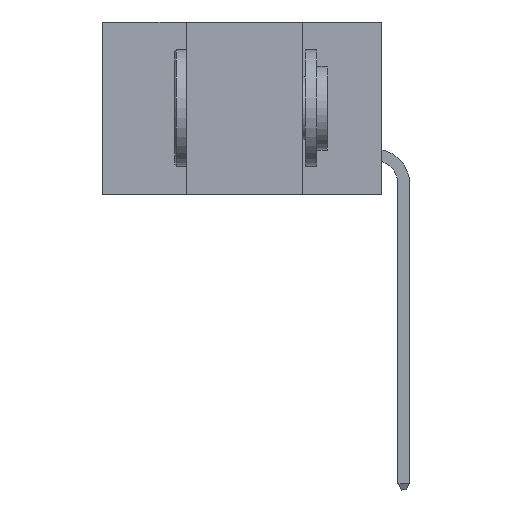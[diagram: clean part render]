
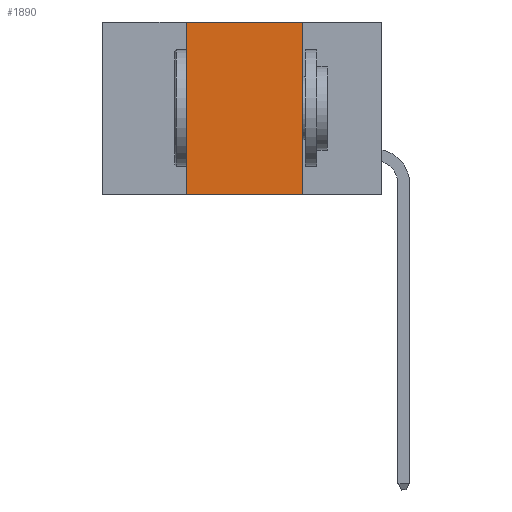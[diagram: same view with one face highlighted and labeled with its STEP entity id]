
A CAD part, left-side view. The second image highlights one B-rep face of the part: STEP entity #1890.
In plain terms, the highlighted planar face has unit normal (-1, 0, 0).
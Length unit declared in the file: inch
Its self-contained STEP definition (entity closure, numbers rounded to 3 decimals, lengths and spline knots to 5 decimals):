
#1890 = ADVANCED_FACE ( 'NONE', ( #22624 ), #2279, .F. ) ;
#2071 = EDGE_CURVE ( 'NONE', #20057, #4016, #4633, .T. ) ;
#2279 = PLANE ( 'NONE',  #12350 ) ;
#2307 = VECTOR ( 'NONE', #10047, 39.37008 ) ;
#2604 = EDGE_CURVE ( 'NONE', #4016, #10516, #32461, .T. ) ;
#4016 = VERTEX_POINT ( 'NONE', #5179 ) ;
#4633 = LINE ( 'NONE', #22464, #2307 ) ;
#4863 = DIRECTION ( 'NONE',  ( 1., 0., 0. ) ) ;
#4964 = CARTESIAN_POINT ( 'NONE',  ( 0., 0.17, -0.37 ) ) ;
#5179 = CARTESIAN_POINT ( 'NONE',  ( 0., 0.42, 0. ) ) ;
#5896 = ORIENTED_EDGE ( 'NONE', *, *, #2604, .F. ) ;
#6288 = VECTOR ( 'NONE', #30094, 39.37008 ) ;
#6990 = CARTESIAN_POINT ( 'NONE',  ( 0., 0.17, 0. ) ) ;
#9812 = CARTESIAN_POINT ( 'NONE',  ( 0., 0.6, 0. ) ) ;
#9874 = ORIENTED_EDGE ( 'NONE', *, *, #2071, .F. ) ;
#10047 = DIRECTION ( 'NONE',  ( 0., 0., 1. ) ) ;
#10161 = CARTESIAN_POINT ( 'NONE',  ( 0., 0.42, -0.37 ) ) ;
#10516 = VERTEX_POINT ( 'NONE', #29559 ) ;
#12350 = AXIS2_PLACEMENT_3D ( 'NONE', #27104, #4863, #29752 ) ;
#13714 = EDGE_CURVE ( 'NONE', #10516, #28076, #28216, .T. ) ;
#14443 = DIRECTION ( 'NONE',  ( 0., 0., -1. ) ) ;
#14990 = CARTESIAN_POINT ( 'NONE',  ( 0., 0.6, -0.37 ) ) ;
#16266 = ORIENTED_EDGE ( 'NONE', *, *, #17710, .T. ) ;
#17710 = EDGE_CURVE ( 'NONE', #20057, #28076, #24316, .T. ) ;
#18208 = VECTOR ( 'NONE', #32276, 39.37008 ) ;
#20057 = VERTEX_POINT ( 'NONE', #10161 ) ;
#22464 = CARTESIAN_POINT ( 'NONE',  ( 0., 0.42, 0. ) ) ;
#22624 = FACE_OUTER_BOUND ( 'NONE', #25035, .T. ) ;
#24316 = LINE ( 'NONE', #14990, #6288 ) ;
#25035 = EDGE_LOOP ( 'NONE', ( #32175, #5896, #9874, #16266 ) ) ;
#27104 = CARTESIAN_POINT ( 'NONE',  ( 0., 0.6, 0. ) ) ;
#28076 = VERTEX_POINT ( 'NONE', #4964 ) ;
#28216 = LINE ( 'NONE', #6990, #30163 ) ;
#29559 = CARTESIAN_POINT ( 'NONE',  ( 0., 0.17, 0. ) ) ;
#29752 = DIRECTION ( 'NONE',  ( 0., 0., -1. ) ) ;
#30094 = DIRECTION ( 'NONE',  ( 0., -1., 0. ) ) ;
#30163 = VECTOR ( 'NONE', #14443, 39.37008 ) ;
#32175 = ORIENTED_EDGE ( 'NONE', *, *, #13714, .F. ) ;
#32276 = DIRECTION ( 'NONE',  ( 0., -1., 0. ) ) ;
#32461 = LINE ( 'NONE', #9812, #18208 ) ;
